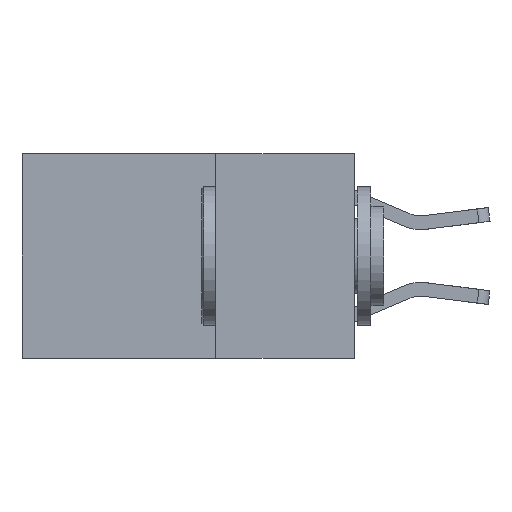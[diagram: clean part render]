
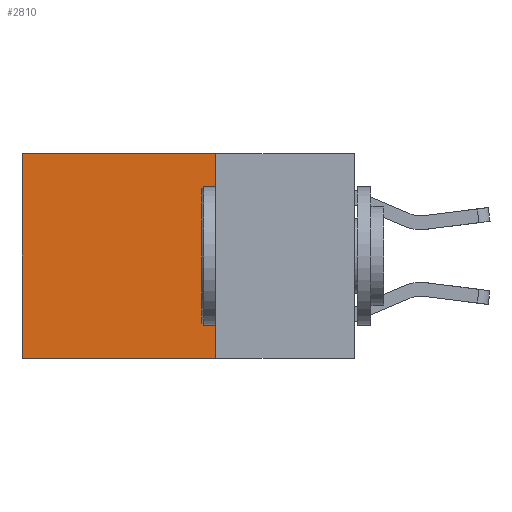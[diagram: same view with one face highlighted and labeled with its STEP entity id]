
A CAD part, left-side view. The second image highlights one B-rep face of the part: STEP entity #2810.
In plain terms, the highlighted planar face has unit normal (-1, 0, 0).
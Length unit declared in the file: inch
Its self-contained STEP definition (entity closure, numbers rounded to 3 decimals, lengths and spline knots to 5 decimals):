
#72 = LINE ( 'NONE', #3661, #8946 ) ;
#142 = ORIENTED_EDGE ( 'NONE', *, *, #5735, .F. ) ;
#422 = DIRECTION ( 'NONE',  ( 0., 0., -1. ) ) ;
#480 = DIRECTION ( 'NONE',  ( 1., 0., 0. ) ) ;
#651 = PLANE ( 'NONE',  #8302 ) ;
#769 = EDGE_CURVE ( 'NONE', #4053, #7360, #1344, .T. ) ;
#784 = CARTESIAN_POINT ( 'NONE',  ( 0.2625, 0.25, 0. ) ) ;
#910 = CARTESIAN_POINT ( 'NONE',  ( 0.2625, 0.6, -0.37 ) ) ;
#1344 = LINE ( 'NONE', #1943, #9905 ) ;
#1524 = CARTESIAN_POINT ( 'NONE',  ( 0.2625, 0.25, 0. ) ) ;
#1531 = DIRECTION ( 'NONE',  ( 0., 1., 0. ) ) ;
#1845 = LINE ( 'NONE', #1524, #3942 ) ;
#1943 = CARTESIAN_POINT ( 'NONE',  ( 0.2625, 0.25, 0. ) ) ;
#2050 = CARTESIAN_POINT ( 'NONE',  ( 0.2625, 0.25, -0.37 ) ) ;
#2088 = EDGE_CURVE ( 'NONE', #7360, #2134, #72, .T. ) ;
#2134 = VERTEX_POINT ( 'NONE', #910 ) ;
#2169 = LINE ( 'NONE', #6360, #6295 ) ;
#2255 = ORIENTED_EDGE ( 'NONE', *, *, #769, .T. ) ;
#2317 = DIRECTION ( 'NONE',  ( 0., 0., -1. ) ) ;
#2810 = ADVANCED_FACE ( 'NONE', ( #6028 ), #651, .F. ) ;
#3661 = CARTESIAN_POINT ( 'NONE',  ( 0.2625, 0.6, 0. ) ) ;
#3942 = VECTOR ( 'NONE', #2317, 39.37008 ) ;
#4053 = VERTEX_POINT ( 'NONE', #7073 ) ;
#4198 = EDGE_LOOP ( 'NONE', ( #4444, #8763, #142, #2255 ) ) ;
#4444 = ORIENTED_EDGE ( 'NONE', *, *, #2088, .T. ) ;
#5735 = EDGE_CURVE ( 'NONE', #4053, #8060, #1845, .T. ) ;
#5783 = CARTESIAN_POINT ( 'NONE',  ( 0.2625, 0.6, 0. ) ) ;
#6028 = FACE_OUTER_BOUND ( 'NONE', #4198, .T. ) ;
#6295 = VECTOR ( 'NONE', #7946, 39.37008 ) ;
#6360 = CARTESIAN_POINT ( 'NONE',  ( 0.2625, 0.25, -0.37 ) ) ;
#6434 = DIRECTION ( 'NONE',  ( 0., 0., -1. ) ) ;
#7073 = CARTESIAN_POINT ( 'NONE',  ( 0.2625, 0.25, 0. ) ) ;
#7360 = VERTEX_POINT ( 'NONE', #5783 ) ;
#7946 = DIRECTION ( 'NONE',  ( 0., 1., 0. ) ) ;
#8060 = VERTEX_POINT ( 'NONE', #2050 ) ;
#8302 = AXIS2_PLACEMENT_3D ( 'NONE', #784, #480, #422 ) ;
#8763 = ORIENTED_EDGE ( 'NONE', *, *, #9832, .F. ) ;
#8946 = VECTOR ( 'NONE', #6434, 39.37008 ) ;
#9832 = EDGE_CURVE ( 'NONE', #8060, #2134, #2169, .T. ) ;
#9905 = VECTOR ( 'NONE', #1531, 39.37008 ) ;
